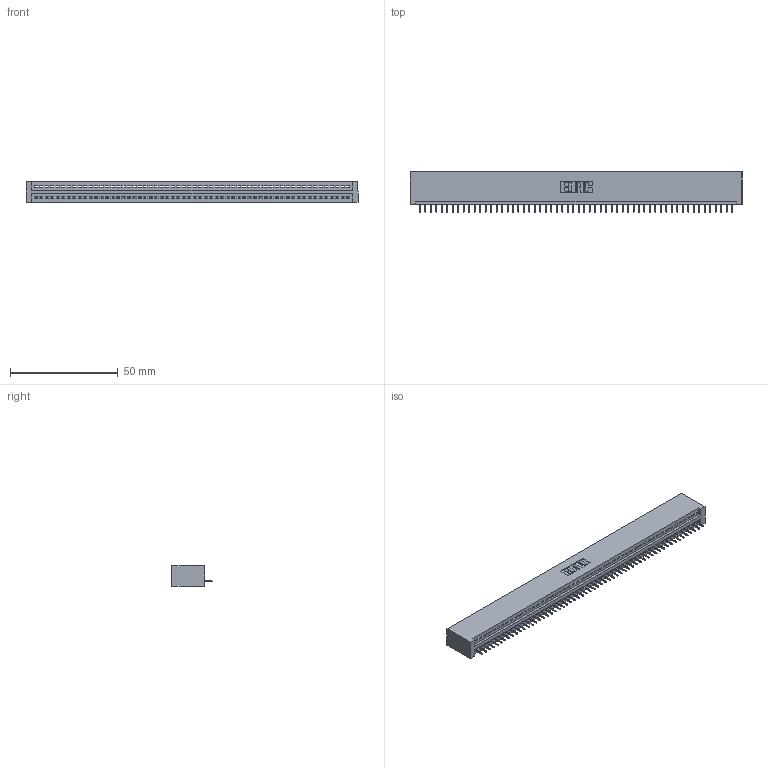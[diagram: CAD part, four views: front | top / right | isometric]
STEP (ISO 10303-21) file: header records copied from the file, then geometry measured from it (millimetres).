
FILE_DESCRIPTION (( 'STEP AP203' ), '1' );
FILE_NAME ('395-058-525-101.STEP', '2020-09-24T18:19:14', ( '' ), ( '' ), 'SwSTEP 2.0', 'SolidWorks 2020', '' );
FILE_SCHEMA (( 'CONFIG_CONTROL_DESIGN' ));
Length unit declared in the file: inch
Products named in the file (3): 345 Part_No Mounting Lugs; 345-292-001_345-293-125; 395-058-525-101
Assembly tree (59 placements, depth 2):
  395-058-525-101
    345 Part_No Mounting Lugs
    345-292-001_345-293-125  x58
Bounding box: 153.92 x 18.72 x 9.4 mm (x, y, z)
Volume: 15098.5 mm3; surface area: 19682.4 mm2
Topology: 59 solids, 59 shells, 3714 faces, 10757 edges, 6938 vertices
Faces by surface type: plane 2744, cylinder 970
Entity records: 41295 total; most frequent: CARTESIAN_POINT 7158, ORIENTED_EDGE 7150, DIRECTION 6223, EDGE_CURVE 3575, VECTOR 3223, LINE 3223, VERTEX_POINT 2378, AXIS2_PLACEMENT_3D 1500
